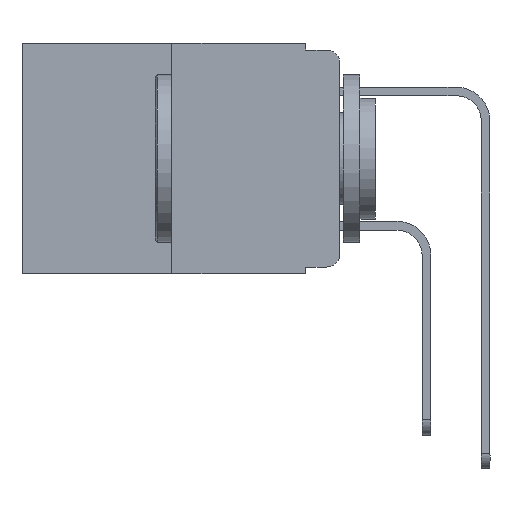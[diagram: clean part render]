
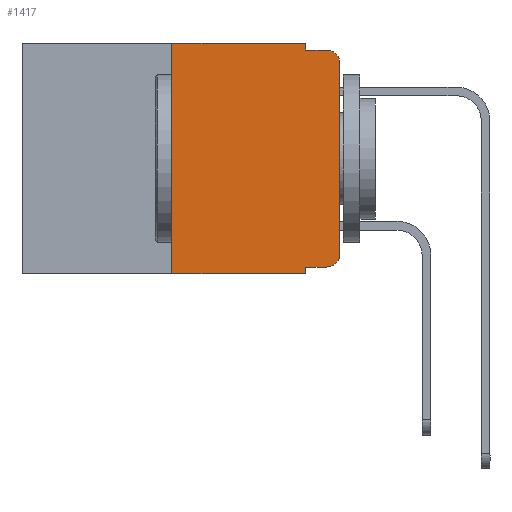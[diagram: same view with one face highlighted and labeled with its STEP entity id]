
A CAD part, left-side view. The second image highlights one B-rep face of the part: STEP entity #1417.
In plain terms, the highlighted planar face has unit normal (-1, 0, 0).
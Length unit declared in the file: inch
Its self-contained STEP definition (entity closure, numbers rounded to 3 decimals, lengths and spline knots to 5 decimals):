
#301 = ORIENTED_EDGE ( 'NONE', *, *, #6907, .T. ) ;
#650 = VECTOR ( 'NONE', #26178, 39.37008 ) ;
#779 = CARTESIAN_POINT ( 'NONE',  ( 0., 0.25, -0.343 ) ) ;
#892 = DIRECTION ( 'NONE',  ( 1., 0., 0. ) ) ;
#899 = CARTESIAN_POINT ( 'NONE',  ( 0., 0.051, -0.01 ) ) ;
#981 = CARTESIAN_POINT ( 'NONE',  ( 0., 0., 0. ) ) ;
#1126 = AXIS2_PLACEMENT_3D ( 'NONE', #6873, #10652, #2651 ) ;
#1417 = ADVANCED_FACE ( 'NONE', ( #11488 ), #3081, .F. ) ;
#2651 = DIRECTION ( 'NONE',  ( 0., 0., -1. ) ) ;
#3037 = CARTESIAN_POINT ( 'NONE',  ( 0., 0.051, -0.333 ) ) ;
#3081 = PLANE ( 'NONE',  #14046 ) ;
#3099 = EDGE_CURVE ( 'NONE', #6735, #21345, #25733, .T. ) ;
#3336 = VECTOR ( 'NONE', #6998, 39.37008 ) ;
#3460 = CARTESIAN_POINT ( 'NONE',  ( 0., 0.051, 0. ) ) ;
#3476 = CARTESIAN_POINT ( 'NONE',  ( 0., 0.051, -0.333 ) ) ;
#4686 = DIRECTION ( 'NONE',  ( 0., 0., -1. ) ) ;
#4699 = CIRCLE ( 'NONE', #23755, 0.02 ) ;
#5091 = VECTOR ( 'NONE', #19189, 39.37008 ) ;
#5294 = EDGE_CURVE ( 'NONE', #7965, #6735, #5758, .T. ) ;
#5352 = VERTEX_POINT ( 'NONE', #3476 ) ;
#5758 = LINE ( 'NONE', #26688, #17434 ) ;
#5825 = CARTESIAN_POINT ( 'NONE',  ( 0., 0., -0.313 ) ) ;
#5851 = CARTESIAN_POINT ( 'NONE',  ( 0., 0.051, -0.343 ) ) ;
#5968 = ORIENTED_EDGE ( 'NONE', *, *, #5294, .F. ) ;
#6224 = EDGE_CURVE ( 'NONE', #20619, #8765, #4699, .T. ) ;
#6712 = LINE ( 'NONE', #23651, #5091 ) ;
#6735 = VERTEX_POINT ( 'NONE', #14604 ) ;
#6873 = CARTESIAN_POINT ( 'NONE',  ( 0., 0.02, -0.03 ) ) ;
#6907 = EDGE_CURVE ( 'NONE', #8765, #11000, #7124, .T. ) ;
#6998 = DIRECTION ( 'NONE',  ( 0., 0., 1. ) ) ;
#7124 = LINE ( 'NONE', #981, #3336 ) ;
#7965 = VERTEX_POINT ( 'NONE', #11122 ) ;
#8765 = VERTEX_POINT ( 'NONE', #5825 ) ;
#10016 = CARTESIAN_POINT ( 'NONE',  ( 0., 0.051, -0.01 ) ) ;
#10107 = VERTEX_POINT ( 'NONE', #5851 ) ;
#10148 = CARTESIAN_POINT ( 'NONE',  ( 0., 0.02, -0.313 ) ) ;
#10289 = VECTOR ( 'NONE', #21554, 39.37008 ) ;
#10652 = DIRECTION ( 'NONE',  ( -1., 0., 0. ) ) ;
#11000 = VERTEX_POINT ( 'NONE', #26680 ) ;
#11122 = CARTESIAN_POINT ( 'NONE',  ( 0., 0.25, 0. ) ) ;
#11356 = CARTESIAN_POINT ( 'NONE',  ( 0., 0.473, 0. ) ) ;
#11488 = FACE_OUTER_BOUND ( 'NONE', #12977, .T. ) ;
#12333 = EDGE_CURVE ( 'NONE', #21700, #7965, #24127, .T. ) ;
#12650 = CARTESIAN_POINT ( 'NONE',  ( 0., 0.02, -0.333 ) ) ;
#12977 = EDGE_LOOP ( 'NONE', ( #301, #26228, #18662, #26686, #5968, #19602, #22364, #21137, #26241, #24168 ) ) ;
#13421 = LINE ( 'NONE', #899, #10289 ) ;
#13978 = EDGE_CURVE ( 'NONE', #11000, #17713, #24121, .T. ) ;
#14046 = AXIS2_PLACEMENT_3D ( 'NONE', #11356, #892, #19637 ) ;
#14604 = CARTESIAN_POINT ( 'NONE',  ( 0., 0.051, 0. ) ) ;
#16382 = DIRECTION ( 'NONE',  ( 0., -1., 0. ) ) ;
#16965 = EDGE_CURVE ( 'NONE', #21700, #10107, #6712, .T. ) ;
#17160 = CARTESIAN_POINT ( 'NONE',  ( 0., 0.02, -0.01 ) ) ;
#17434 = VECTOR ( 'NONE', #16382, 39.37008 ) ;
#17448 = EDGE_CURVE ( 'NONE', #5352, #10107, #20287, .T. ) ;
#17713 = VERTEX_POINT ( 'NONE', #17160 ) ;
#18207 = VECTOR ( 'NONE', #4686, 39.37008 ) ;
#18662 = ORIENTED_EDGE ( 'NONE', *, *, #26603, .F. ) ;
#19046 = EDGE_CURVE ( 'NONE', #5352, #20619, #23789, .T. ) ;
#19189 = DIRECTION ( 'NONE',  ( 0., -1., 0. ) ) ;
#19602 = ORIENTED_EDGE ( 'NONE', *, *, #12333, .F. ) ;
#19637 = DIRECTION ( 'NONE',  ( 0., 0., -1. ) ) ;
#19859 = DIRECTION ( 'NONE',  ( 0., -1., 0. ) ) ;
#20287 = LINE ( 'NONE', #3460, #26380 ) ;
#20476 = DIRECTION ( 'NONE',  ( -1., 0., 0. ) ) ;
#20619 = VERTEX_POINT ( 'NONE', #12650 ) ;
#21137 = ORIENTED_EDGE ( 'NONE', *, *, #17448, .F. ) ;
#21345 = VERTEX_POINT ( 'NONE', #10016 ) ;
#21554 = DIRECTION ( 'NONE',  ( 0., -1., 0. ) ) ;
#21700 = VERTEX_POINT ( 'NONE', #779 ) ;
#22364 = ORIENTED_EDGE ( 'NONE', *, *, #16965, .T. ) ;
#22371 = CARTESIAN_POINT ( 'NONE',  ( 0., 0.25, 0. ) ) ;
#23651 = CARTESIAN_POINT ( 'NONE',  ( 0., 0.473, -0.343 ) ) ;
#23755 = AXIS2_PLACEMENT_3D ( 'NONE', #10148, #20476, #26725 ) ;
#23789 = LINE ( 'NONE', #3037, #26024 ) ;
#24077 = DIRECTION ( 'NONE',  ( 0., 0., -1. ) ) ;
#24121 = CIRCLE ( 'NONE', #1126, 0.02 ) ;
#24127 = LINE ( 'NONE', #22371, #650 ) ;
#24168 = ORIENTED_EDGE ( 'NONE', *, *, #6224, .T. ) ;
#25608 = CARTESIAN_POINT ( 'NONE',  ( 0., 0.051, 0. ) ) ;
#25733 = LINE ( 'NONE', #25608, #18207 ) ;
#26024 = VECTOR ( 'NONE', #19859, 39.37008 ) ;
#26178 = DIRECTION ( 'NONE',  ( 0., 0., 1. ) ) ;
#26228 = ORIENTED_EDGE ( 'NONE', *, *, #13978, .T. ) ;
#26241 = ORIENTED_EDGE ( 'NONE', *, *, #19046, .T. ) ;
#26380 = VECTOR ( 'NONE', #24077, 39.37008 ) ;
#26603 = EDGE_CURVE ( 'NONE', #21345, #17713, #13421, .T. ) ;
#26680 = CARTESIAN_POINT ( 'NONE',  ( 0., 0., -0.03 ) ) ;
#26686 = ORIENTED_EDGE ( 'NONE', *, *, #3099, .F. ) ;
#26688 = CARTESIAN_POINT ( 'NONE',  ( 0., 0.473, 0. ) ) ;
#26725 = DIRECTION ( 'NONE',  ( 0., 0., -1. ) ) ;
